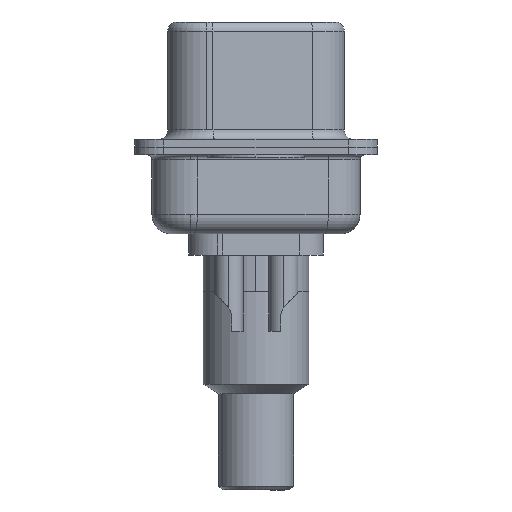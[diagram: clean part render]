
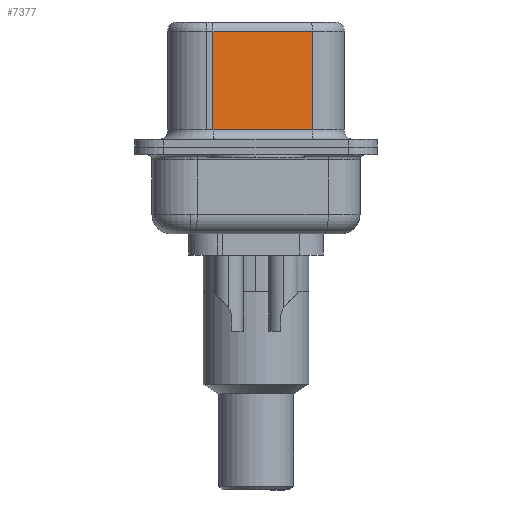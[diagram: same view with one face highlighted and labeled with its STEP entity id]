
A CAD part, left-side view. The second image highlights one B-rep face of the part: STEP entity #7377.
In plain terms, the highlighted planar face has unit normal (-0.985, -0.174, 0).
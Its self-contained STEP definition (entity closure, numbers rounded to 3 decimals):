
#204 = EDGE_LOOP ( 'NONE', ( #16312, #13745, #13405, #8278 ) ) ;
#400 = EDGE_CURVE ( 'NONE', #12631, #7096, #14155, .T. ) ;
#452 = LINE ( 'NONE', #14928, #3842 ) ;
#3842 = VECTOR ( 'NONE', #6710, 1000. ) ;
#4601 = EDGE_CURVE ( 'NONE', #15990, #7862, #452, .T. ) ;
#4846 = DIRECTION ( 'NONE',  ( 0.174, -0.985, 0. ) ) ;
#4910 = AXIS2_PLACEMENT_3D ( 'NONE', #8410, #5589, #15559 ) ;
#5126 = CARTESIAN_POINT ( 'NONE',  ( 4.565, -2.927, 0.9 ) ) ;
#5468 = VECTOR ( 'NONE', #10862, 1000. ) ;
#5589 = DIRECTION ( 'NONE',  ( 0.985, 0.174, 0. ) ) ;
#6710 = DIRECTION ( 'NONE',  ( 0., 0., -1. ) ) ;
#7096 = VERTEX_POINT ( 'NONE', #14940 ) ;
#7377 = ADVANCED_FACE ( 'NONE', ( #16765 ), #14101, .F. ) ;
#7707 = DIRECTION ( 'NONE',  ( 0., 0., -1. ) ) ;
#7862 = VERTEX_POINT ( 'NONE', #5126 ) ;
#8278 = ORIENTED_EDGE ( 'NONE', *, *, #15043, .T. ) ;
#8410 = CARTESIAN_POINT ( 'NONE',  ( 4.565, -2.927, 6.52 ) ) ;
#8777 = VECTOR ( 'NONE', #4846, 1000. ) ;
#9221 = LINE ( 'NONE', #13392, #8777 ) ;
#9705 = LINE ( 'NONE', #17972, #5468 ) ;
#10862 = DIRECTION ( 'NONE',  ( -0.174, 0.985, 0. ) ) ;
#12631 = VERTEX_POINT ( 'NONE', #17734 ) ;
#13253 = VECTOR ( 'NONE', #7707, 1000. ) ;
#13333 = EDGE_CURVE ( 'NONE', #15990, #12631, #9705, .T. ) ;
#13392 = CARTESIAN_POINT ( 'NONE',  ( 4.565, -2.927, 0.9 ) ) ;
#13405 = ORIENTED_EDGE ( 'NONE', *, *, #400, .T. ) ;
#13745 = ORIENTED_EDGE ( 'NONE', *, *, #13333, .T. ) ;
#14101 = PLANE ( 'NONE',  #4910 ) ;
#14155 = LINE ( 'NONE', #18342, #13253 ) ;
#14928 = CARTESIAN_POINT ( 'NONE',  ( 4.565, -2.927, 6.52 ) ) ;
#14940 = CARTESIAN_POINT ( 'NONE',  ( 3.655, 2.233, 0.9 ) ) ;
#15043 = EDGE_CURVE ( 'NONE', #7096, #7862, #9221, .T. ) ;
#15559 = DIRECTION ( 'NONE',  ( -0.174, 0.985, 0. ) ) ;
#15990 = VERTEX_POINT ( 'NONE', #17541 ) ;
#16312 = ORIENTED_EDGE ( 'NONE', *, *, #4601, .F. ) ;
#16765 = FACE_OUTER_BOUND ( 'NONE', #204, .T. ) ;
#17541 = CARTESIAN_POINT ( 'NONE',  ( 4.565, -2.927, 6.02 ) ) ;
#17734 = CARTESIAN_POINT ( 'NONE',  ( 3.655, 2.233, 6.02 ) ) ;
#17972 = CARTESIAN_POINT ( 'NONE',  ( 4.565, -2.927, 6.02 ) ) ;
#18342 = CARTESIAN_POINT ( 'NONE',  ( 3.655, 2.233, 6.52 ) ) ;
